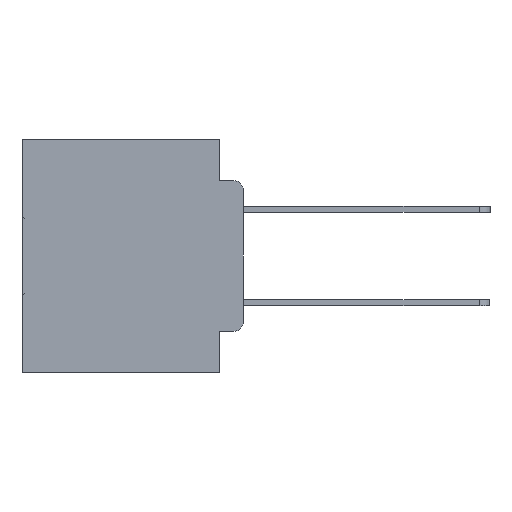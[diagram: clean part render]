
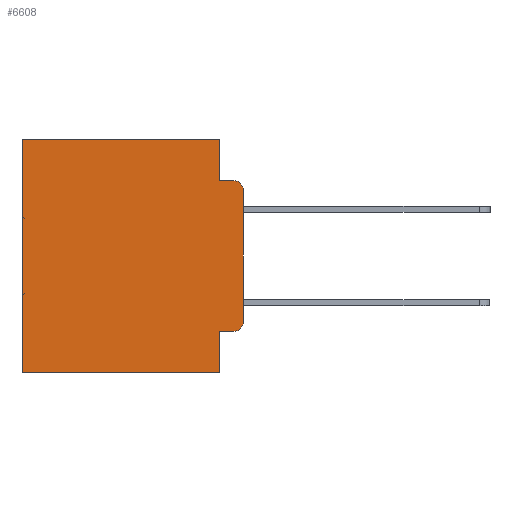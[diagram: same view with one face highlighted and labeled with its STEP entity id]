
A CAD part, left-side view. The second image highlights one B-rep face of the part: STEP entity #6608.
In plain terms, the highlighted planar face has unit normal (-1, 0, 0).
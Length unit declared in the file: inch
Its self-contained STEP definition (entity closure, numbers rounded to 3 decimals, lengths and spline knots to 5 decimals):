
#141 = CIRCLE ( 'NONE', #1929, 0.02 ) ;
#245 = ORIENTED_EDGE ( 'NONE', *, *, #18237, .T. ) ;
#391 = VECTOR ( 'NONE', #27930, 39.37008 ) ;
#1311 = DIRECTION ( 'NONE',  ( 0., 1., 0. ) ) ;
#1488 = DIRECTION ( 'NONE',  ( 0., 0., -1. ) ) ;
#1532 = DIRECTION ( 'NONE',  ( 0., -1., 0. ) ) ;
#1929 = AXIS2_PLACEMENT_3D ( 'NONE', #14895, #33188, #17571 ) ;
#4084 = VERTEX_POINT ( 'NONE', #13054 ) ;
#4415 = CARTESIAN_POINT ( 'NONE',  ( 0.298, 0.051, -0.4115 ) ) ;
#4484 = ORIENTED_EDGE ( 'NONE', *, *, #16927, .F. ) ;
#4598 = DIRECTION ( 'NONE',  ( -1., 0., 0. ) ) ;
#4797 = CARTESIAN_POINT ( 'NONE',  ( 0.298, 0.051, -0.4115 ) ) ;
#5412 = VERTEX_POINT ( 'NONE', #23185 ) ;
#5712 = CARTESIAN_POINT ( 'NONE',  ( 0.298, 0.473, -0.5 ) ) ;
#6120 = CARTESIAN_POINT ( 'NONE',  ( 0.298, 0., 0. ) ) ;
#6608 = ADVANCED_FACE ( 'NONE', ( #27288 ), #30711, .F. ) ;
#6644 = CARTESIAN_POINT ( 'NONE',  ( 0.298, 0.02, -0.4115 ) ) ;
#7541 = AXIS2_PLACEMENT_3D ( 'NONE', #20592, #4598, #23240 ) ;
#7938 = EDGE_CURVE ( 'NONE', #27710, #13703, #13165, .T. ) ;
#8509 = CARTESIAN_POINT ( 'NONE',  ( 0.298, 0.051, -0.5 ) ) ;
#9921 = ORIENTED_EDGE ( 'NONE', *, *, #29239, .T. ) ;
#10316 = CARTESIAN_POINT ( 'NONE',  ( 0.298, 0., -0.3915 ) ) ;
#11074 = VERTEX_POINT ( 'NONE', #10316 ) ;
#12137 = CARTESIAN_POINT ( 'NONE',  ( 0.298, 0.051, 0. ) ) ;
#12398 = CARTESIAN_POINT ( 'NONE',  ( 0.298, 0.473, 0. ) ) ;
#12406 = DIRECTION ( 'NONE',  ( 0., 0., -1. ) ) ;
#12978 = VERTEX_POINT ( 'NONE', #16333 ) ;
#13054 = CARTESIAN_POINT ( 'NONE',  ( 0.298, 0.051, 0. ) ) ;
#13165 = LINE ( 'NONE', #30576, #19430 ) ;
#13703 = VERTEX_POINT ( 'NONE', #5712 ) ;
#14017 = EDGE_CURVE ( 'NONE', #25167, #27710, #24892, .T. ) ;
#14121 = CIRCLE ( 'NONE', #7541, 0.02 ) ;
#14400 = LINE ( 'NONE', #4797, #15228 ) ;
#14493 = EDGE_CURVE ( 'NONE', #12978, #11074, #24863, .T. ) ;
#14895 = CARTESIAN_POINT ( 'NONE',  ( 0.298, 0.02, -0.1085 ) ) ;
#14992 = ORIENTED_EDGE ( 'NONE', *, *, #19378, .T. ) ;
#15228 = VECTOR ( 'NONE', #20815, 39.37008 ) ;
#15661 = CARTESIAN_POINT ( 'NONE',  ( 0.298, 0.051, -0.0885 ) ) ;
#16333 = CARTESIAN_POINT ( 'NONE',  ( 0.298, 0., -0.1085 ) ) ;
#16912 = EDGE_LOOP ( 'NONE', ( #22414, #9921, #4484, #32580, #33396, #14992, #23651, #19161, #19982, #245 ) ) ;
#16927 = EDGE_CURVE ( 'NONE', #22589, #5412, #22101, .T. ) ;
#17030 = LINE ( 'NONE', #21163, #30171 ) ;
#17212 = DIRECTION ( 'NONE',  ( 1., 0., 0. ) ) ;
#17571 = DIRECTION ( 'NONE',  ( 0., 0., -1. ) ) ;
#17658 = CARTESIAN_POINT ( 'NONE',  ( 0.298, 0.473, 0. ) ) ;
#18237 = EDGE_CURVE ( 'NONE', #30948, #11074, #14121, .T. ) ;
#18371 = EDGE_CURVE ( 'NONE', #4084, #19390, #17030, .T. ) ;
#18794 = VECTOR ( 'NONE', #12406, 39.37008 ) ;
#19161 = ORIENTED_EDGE ( 'NONE', *, *, #14017, .F. ) ;
#19378 = EDGE_CURVE ( 'NONE', #19390, #13703, #22338, .T. ) ;
#19390 = VERTEX_POINT ( 'NONE', #12398 ) ;
#19430 = VECTOR ( 'NONE', #1311, 39.37008 ) ;
#19982 = ORIENTED_EDGE ( 'NONE', *, *, #30527, .T. ) ;
#20592 = CARTESIAN_POINT ( 'NONE',  ( 0.298, 0.02, -0.3915 ) ) ;
#20815 = DIRECTION ( 'NONE',  ( 0., -1., 0. ) ) ;
#20942 = LINE ( 'NONE', #12137, #391 ) ;
#21163 = CARTESIAN_POINT ( 'NONE',  ( 0.298, 0., 0. ) ) ;
#22101 = LINE ( 'NONE', #33250, #29053 ) ;
#22123 = DIRECTION ( 'NONE',  ( 0., 0., -1. ) ) ;
#22338 = LINE ( 'NONE', #17658, #28449 ) ;
#22414 = ORIENTED_EDGE ( 'NONE', *, *, #14493, .F. ) ;
#22589 = VERTEX_POINT ( 'NONE', #15661 ) ;
#23185 = CARTESIAN_POINT ( 'NONE',  ( 0.298, 0.02, -0.0885 ) ) ;
#23240 = DIRECTION ( 'NONE',  ( 0., 0., -1. ) ) ;
#23651 = ORIENTED_EDGE ( 'NONE', *, *, #7938, .F. ) ;
#24863 = LINE ( 'NONE', #6120, #31807 ) ;
#24892 = LINE ( 'NONE', #28198, #18794 ) ;
#25167 = VERTEX_POINT ( 'NONE', #4415 ) ;
#27288 = FACE_OUTER_BOUND ( 'NONE', #16912, .T. ) ;
#27710 = VERTEX_POINT ( 'NONE', #8509 ) ;
#27930 = DIRECTION ( 'NONE',  ( 0., 0., -1. ) ) ;
#28089 = CARTESIAN_POINT ( 'NONE',  ( 0.298, 0., 0. ) ) ;
#28198 = CARTESIAN_POINT ( 'NONE',  ( 0.298, 0.051, 0. ) ) ;
#28449 = VECTOR ( 'NONE', #33268, 39.37008 ) ;
#28478 = AXIS2_PLACEMENT_3D ( 'NONE', #28089, #17212, #1488 ) ;
#29053 = VECTOR ( 'NONE', #1532, 39.37008 ) ;
#29239 = EDGE_CURVE ( 'NONE', #12978, #5412, #141, .T. ) ;
#30171 = VECTOR ( 'NONE', #31524, 39.37008 ) ;
#30527 = EDGE_CURVE ( 'NONE', #25167, #30948, #14400, .T. ) ;
#30576 = CARTESIAN_POINT ( 'NONE',  ( 0.298, 0., -0.5 ) ) ;
#30711 = PLANE ( 'NONE',  #28478 ) ;
#30948 = VERTEX_POINT ( 'NONE', #6644 ) ;
#31524 = DIRECTION ( 'NONE',  ( 0., 1., 0. ) ) ;
#31611 = EDGE_CURVE ( 'NONE', #4084, #22589, #20942, .T. ) ;
#31807 = VECTOR ( 'NONE', #22123, 39.37008 ) ;
#32580 = ORIENTED_EDGE ( 'NONE', *, *, #31611, .F. ) ;
#33188 = DIRECTION ( 'NONE',  ( -1., 0., 0. ) ) ;
#33250 = CARTESIAN_POINT ( 'NONE',  ( 0.298, 0.051, -0.0885 ) ) ;
#33268 = DIRECTION ( 'NONE',  ( 0., 0., -1. ) ) ;
#33396 = ORIENTED_EDGE ( 'NONE', *, *, #18371, .T. ) ;
